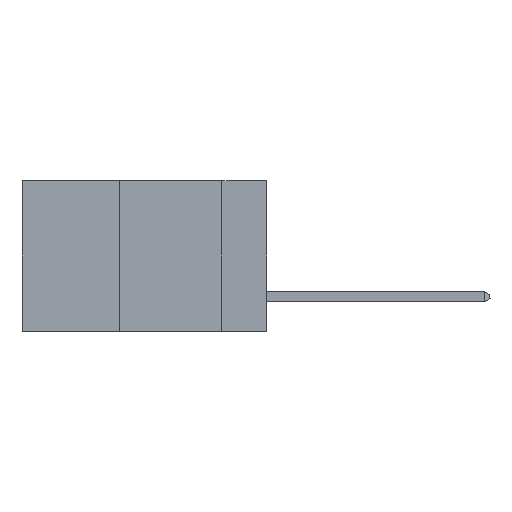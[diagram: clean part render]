
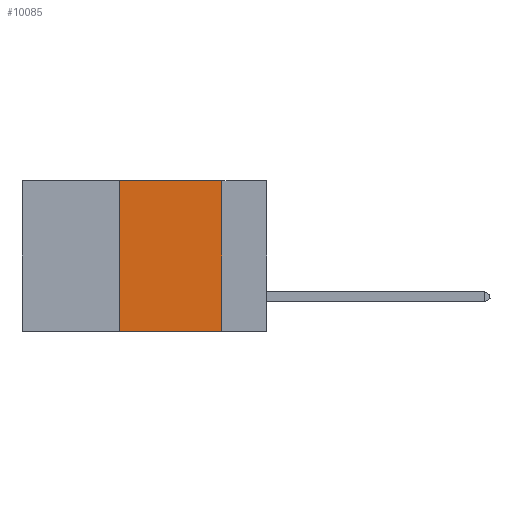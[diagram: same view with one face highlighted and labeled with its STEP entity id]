
A CAD part, left-side view. The second image highlights one B-rep face of the part: STEP entity #10085.
In plain terms, the highlighted planar face has unit normal (-1, 0, 0).
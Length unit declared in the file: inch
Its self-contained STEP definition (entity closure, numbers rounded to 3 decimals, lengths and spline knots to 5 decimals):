
#1102 = CARTESIAN_POINT ( 'NONE',  ( 0., 0.11, -0.37 ) ) ;
#2234 = DIRECTION ( 'NONE',  ( 0., -1., 0. ) ) ;
#2539 = EDGE_CURVE ( 'NONE', #13804, #11927, #8504, .T. ) ;
#4001 = CARTESIAN_POINT ( 'NONE',  ( 0., 0.36, 0. ) ) ;
#4086 = DIRECTION ( 'NONE',  ( 0., 0., -1. ) ) ;
#4411 = ORIENTED_EDGE ( 'NONE', *, *, #9553, .F. ) ;
#4559 = ORIENTED_EDGE ( 'NONE', *, *, #6384, .F. ) ;
#5821 = DIRECTION ( 'NONE',  ( 0., -1., 0. ) ) ;
#5977 = CARTESIAN_POINT ( 'NONE',  ( 0., 0.36, 0. ) ) ;
#6384 = EDGE_CURVE ( 'NONE', #11927, #18760, #8833, .T. ) ;
#6802 = PLANE ( 'NONE',  #13139 ) ;
#7359 = CARTESIAN_POINT ( 'NONE',  ( 0., 0.6, -0.37 ) ) ;
#7725 = CARTESIAN_POINT ( 'NONE',  ( 0., 0.36, -0.37 ) ) ;
#8504 = LINE ( 'NONE', #16907, #13126 ) ;
#8661 = ORIENTED_EDGE ( 'NONE', *, *, #18675, .T. ) ;
#8833 = LINE ( 'NONE', #13790, #16548 ) ;
#9553 = EDGE_CURVE ( 'NONE', #16364, #13804, #14621, .T. ) ;
#10018 = EDGE_LOOP ( 'NONE', ( #4559, #13483, #4411, #8661 ) ) ;
#10085 = ADVANCED_FACE ( 'NONE', ( #10465 ), #6802, .F. ) ;
#10465 = FACE_OUTER_BOUND ( 'NONE', #10018, .T. ) ;
#11692 = DIRECTION ( 'NONE',  ( 0., 0., -1. ) ) ;
#11899 = LINE ( 'NONE', #7359, #15232 ) ;
#11927 = VERTEX_POINT ( 'NONE', #16746 ) ;
#13126 = VECTOR ( 'NONE', #2234, 39.37008 ) ;
#13139 = AXIS2_PLACEMENT_3D ( 'NONE', #18335, #19830, #11692 ) ;
#13483 = ORIENTED_EDGE ( 'NONE', *, *, #2539, .F. ) ;
#13790 = CARTESIAN_POINT ( 'NONE',  ( 0., 0.11, 0. ) ) ;
#13804 = VERTEX_POINT ( 'NONE', #5977 ) ;
#14621 = LINE ( 'NONE', #4001, #18460 ) ;
#15232 = VECTOR ( 'NONE', #5821, 39.37008 ) ;
#16364 = VERTEX_POINT ( 'NONE', #7725 ) ;
#16548 = VECTOR ( 'NONE', #4086, 39.37008 ) ;
#16746 = CARTESIAN_POINT ( 'NONE',  ( 0., 0.11, 0. ) ) ;
#16907 = CARTESIAN_POINT ( 'NONE',  ( 0., 0.6, 0. ) ) ;
#18335 = CARTESIAN_POINT ( 'NONE',  ( 0., 0.6, 0. ) ) ;
#18460 = VECTOR ( 'NONE', #20145, 39.37008 ) ;
#18675 = EDGE_CURVE ( 'NONE', #16364, #18760, #11899, .T. ) ;
#18760 = VERTEX_POINT ( 'NONE', #1102 ) ;
#19830 = DIRECTION ( 'NONE',  ( 1., 0., 0. ) ) ;
#20145 = DIRECTION ( 'NONE',  ( 0., 0., 1. ) ) ;
